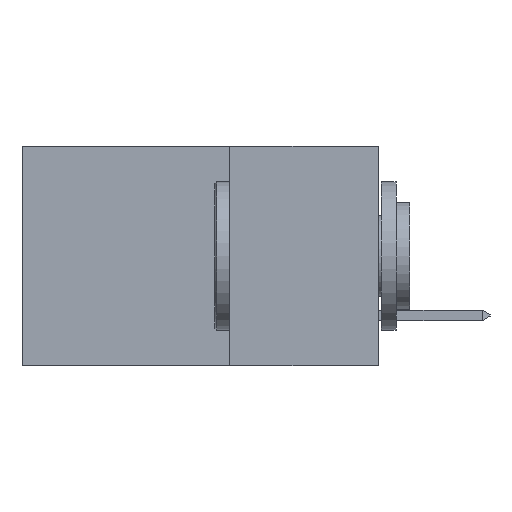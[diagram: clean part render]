
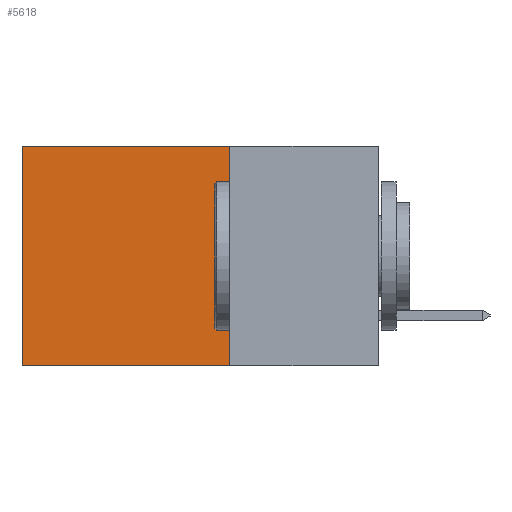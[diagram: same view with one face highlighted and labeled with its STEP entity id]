
A CAD part, left-side view. The second image highlights one B-rep face of the part: STEP entity #5618.
In plain terms, the highlighted planar face has unit normal (-1, 0, 0).
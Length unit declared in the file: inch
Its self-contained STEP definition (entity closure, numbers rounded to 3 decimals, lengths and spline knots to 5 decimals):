
#6 = DIRECTION ( 'NONE',  ( 0., 0., -1. ) ) ;
#182 = DIRECTION ( 'NONE',  ( 1., 0., 0. ) ) ;
#236 = CARTESIAN_POINT ( 'NONE',  ( 0.2615, 0.6, -0.37 ) ) ;
#541 = ORIENTED_EDGE ( 'NONE', *, *, #11734, .F. ) ;
#1255 = CARTESIAN_POINT ( 'NONE',  ( 0.2615, 0.25, -0.37 ) ) ;
#1484 = DIRECTION ( 'NONE',  ( 0., 1., 0. ) ) ;
#1621 = LINE ( 'NONE', #9203, #6546 ) ;
#1737 = LINE ( 'NONE', #8286, #4433 ) ;
#1770 = CARTESIAN_POINT ( 'NONE',  ( 0.2615, 0.25, -0.37 ) ) ;
#2202 = CARTESIAN_POINT ( 'NONE',  ( 0.2615, 0.6, 0. ) ) ;
#2272 = VERTEX_POINT ( 'NONE', #2202 ) ;
#2417 = ORIENTED_EDGE ( 'NONE', *, *, #8183, .F. ) ;
#3113 = VERTEX_POINT ( 'NONE', #4140 ) ;
#3272 = VECTOR ( 'NONE', #5754, 39.37008 ) ;
#3356 = ORIENTED_EDGE ( 'NONE', *, *, #5768, .T. ) ;
#4140 = CARTESIAN_POINT ( 'NONE',  ( 0.2615, 0.25, 0. ) ) ;
#4343 = PLANE ( 'NONE',  #8706 ) ;
#4433 = VECTOR ( 'NONE', #9200, 39.37008 ) ;
#4976 = EDGE_CURVE ( 'NONE', #2272, #5738, #8898, .T. ) ;
#5618 = ADVANCED_FACE ( 'NONE', ( #7743 ), #4343, .F. ) ;
#5738 = VERTEX_POINT ( 'NONE', #11886 ) ;
#5754 = DIRECTION ( 'NONE',  ( 0., 0., -1. ) ) ;
#5768 = EDGE_CURVE ( 'NONE', #3113, #2272, #1621, .T. ) ;
#5838 = LINE ( 'NONE', #1770, #3272 ) ;
#6245 = EDGE_LOOP ( 'NONE', ( #6932, #2417, #541, #3356 ) ) ;
#6424 = VECTOR ( 'NONE', #6, 39.37008 ) ;
#6546 = VECTOR ( 'NONE', #1484, 39.37008 ) ;
#6932 = ORIENTED_EDGE ( 'NONE', *, *, #4976, .T. ) ;
#7193 = DIRECTION ( 'NONE',  ( 0., 0., -1. ) ) ;
#7200 = VERTEX_POINT ( 'NONE', #1255 ) ;
#7743 = FACE_OUTER_BOUND ( 'NONE', #6245, .T. ) ;
#8183 = EDGE_CURVE ( 'NONE', #7200, #5738, #1737, .T. ) ;
#8286 = CARTESIAN_POINT ( 'NONE',  ( 0.2615, 0.25, -0.37 ) ) ;
#8706 = AXIS2_PLACEMENT_3D ( 'NONE', #10890, #182, #7193 ) ;
#8898 = LINE ( 'NONE', #236, #6424 ) ;
#9200 = DIRECTION ( 'NONE',  ( 0., 1., 0. ) ) ;
#9203 = CARTESIAN_POINT ( 'NONE',  ( 0.2615, 0.25, 0. ) ) ;
#10890 = CARTESIAN_POINT ( 'NONE',  ( 0.2615, 0.25, -0.37 ) ) ;
#11734 = EDGE_CURVE ( 'NONE', #3113, #7200, #5838, .T. ) ;
#11886 = CARTESIAN_POINT ( 'NONE',  ( 0.2615, 0.6, -0.37 ) ) ;
